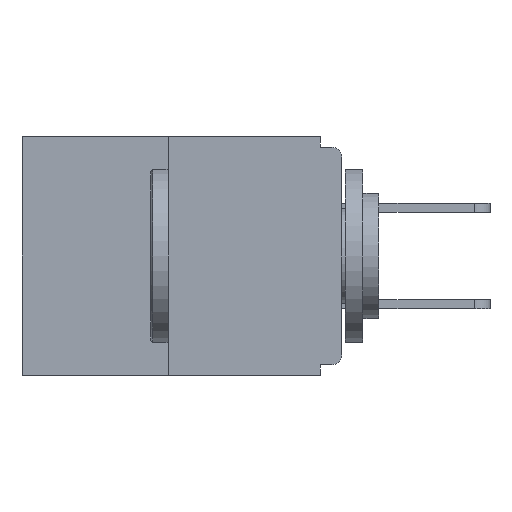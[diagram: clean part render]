
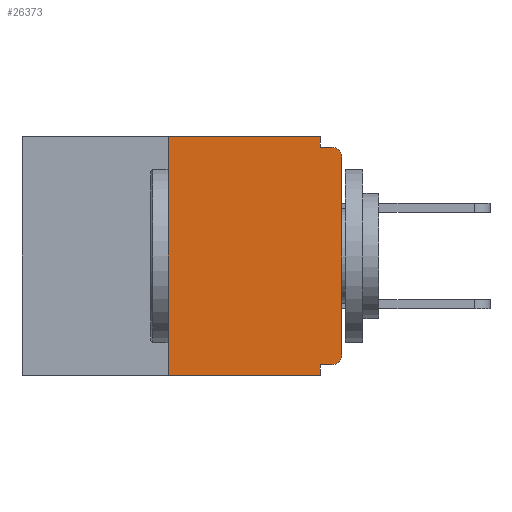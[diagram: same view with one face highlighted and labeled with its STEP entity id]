
A CAD part, left-side view. The second image highlights one B-rep face of the part: STEP entity #26373.
In plain terms, the highlighted planar face has unit normal (-1, 0, 0).
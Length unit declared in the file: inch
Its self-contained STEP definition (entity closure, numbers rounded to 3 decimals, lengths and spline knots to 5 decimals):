
#136 = CARTESIAN_POINT ( 'NONE',  ( 0., 0.031, -0.343 ) ) ;
#201 = CARTESIAN_POINT ( 'NONE',  ( 0., 0.46, 0. ) ) ;
#247 = CIRCLE ( 'NONE', #14551, 0.015 ) ;
#521 = ORIENTED_EDGE ( 'NONE', *, *, #13387, .T. ) ;
#748 = VERTEX_POINT ( 'NONE', #10406 ) ;
#1511 = DIRECTION ( 'NONE',  ( 0., -1., 0. ) ) ;
#1927 = VERTEX_POINT ( 'NONE', #22366 ) ;
#1938 = ORIENTED_EDGE ( 'NONE', *, *, #20720, .T. ) ;
#2018 = VECTOR ( 'NONE', #21718, 39.37008 ) ;
#2052 = LINE ( 'NONE', #16138, #20815 ) ;
#2487 = EDGE_CURVE ( 'NONE', #14383, #1927, #14177, .T. ) ;
#2576 = VERTEX_POINT ( 'NONE', #16046 ) ;
#2694 = ORIENTED_EDGE ( 'NONE', *, *, #5131, .F. ) ;
#2847 = CARTESIAN_POINT ( 'NONE',  ( 0., 0.015, -0.328 ) ) ;
#3844 = DIRECTION ( 'NONE',  ( 0., -1., 0. ) ) ;
#4310 = CARTESIAN_POINT ( 'NONE',  ( 0., 0.46, 0. ) ) ;
#4387 = LINE ( 'NONE', #22350, #19193 ) ;
#4426 = CARTESIAN_POINT ( 'NONE',  ( 0., 0.031, 0. ) ) ;
#5131 = EDGE_CURVE ( 'NONE', #22910, #2576, #16025, .T. ) ;
#5348 = DIRECTION ( 'NONE',  ( -1., 0., 0. ) ) ;
#5556 = CARTESIAN_POINT ( 'NONE',  ( 0., 0.015, -0.03 ) ) ;
#5672 = EDGE_LOOP ( 'NONE', ( #23078, #17036, #1938, #14433, #23446, #25387, #521, #17475, #18691, #2694 ) ) ;
#5759 = DIRECTION ( 'NONE',  ( -1., 0., 0. ) ) ;
#5862 = CARTESIAN_POINT ( 'NONE',  ( 0., 0.46, -0.343 ) ) ;
#6143 = CARTESIAN_POINT ( 'NONE',  ( 0., 0.25, 0. ) ) ;
#6789 = EDGE_CURVE ( 'NONE', #8303, #18234, #25096, .T. ) ;
#8303 = VERTEX_POINT ( 'NONE', #19210 ) ;
#8489 = DIRECTION ( 'NONE',  ( 0., 0., -1. ) ) ;
#8559 = DIRECTION ( 'NONE',  ( 0., 0., 1. ) ) ;
#8616 = VECTOR ( 'NONE', #8559, 39.37008 ) ;
#8622 = VERTEX_POINT ( 'NONE', #14036 ) ;
#9369 = VERTEX_POINT ( 'NONE', #2847 ) ;
#10406 = CARTESIAN_POINT ( 'NONE',  ( 0., 0.031, -0.328 ) ) ;
#11042 = LINE ( 'NONE', #26883, #14306 ) ;
#11385 = FACE_OUTER_BOUND ( 'NONE', #5672, .T. ) ;
#11930 = AXIS2_PLACEMENT_3D ( 'NONE', #201, #12721, #18848 ) ;
#12286 = VECTOR ( 'NONE', #3844, 39.37008 ) ;
#12721 = DIRECTION ( 'NONE',  ( 1., 0., 0. ) ) ;
#13387 = EDGE_CURVE ( 'NONE', #8622, #8303, #11042, .T. ) ;
#14036 = CARTESIAN_POINT ( 'NONE',  ( 0., 0., -0.313 ) ) ;
#14177 = LINE ( 'NONE', #6143, #8616 ) ;
#14306 = VECTOR ( 'NONE', #26518, 39.37008 ) ;
#14383 = VERTEX_POINT ( 'NONE', #14476 ) ;
#14433 = ORIENTED_EDGE ( 'NONE', *, *, #21808, .F. ) ;
#14476 = CARTESIAN_POINT ( 'NONE',  ( 0., 0.25, -0.343 ) ) ;
#14551 = AXIS2_PLACEMENT_3D ( 'NONE', #17958, #5348, #22087 ) ;
#15475 = LINE ( 'NONE', #4310, #26006 ) ;
#15816 = EDGE_CURVE ( 'NONE', #9369, #748, #16798, .T. ) ;
#16025 = LINE ( 'NONE', #4426, #24925 ) ;
#16046 = CARTESIAN_POINT ( 'NONE',  ( 0., 0.031, -0.015 ) ) ;
#16138 = CARTESIAN_POINT ( 'NONE',  ( 0., 0.031, -0.343 ) ) ;
#16158 = VERTEX_POINT ( 'NONE', #136 ) ;
#16798 = LINE ( 'NONE', #17321, #2018 ) ;
#17036 = ORIENTED_EDGE ( 'NONE', *, *, #2487, .F. ) ;
#17279 = DIRECTION ( 'NONE',  ( 0., -1., 0. ) ) ;
#17310 = AXIS2_PLACEMENT_3D ( 'NONE', #5556, #5759, #22383 ) ;
#17321 = CARTESIAN_POINT ( 'NONE',  ( 0., 0., -0.328 ) ) ;
#17475 = ORIENTED_EDGE ( 'NONE', *, *, #6789, .T. ) ;
#17958 = CARTESIAN_POINT ( 'NONE',  ( 0., 0.015, -0.313 ) ) ;
#18234 = VERTEX_POINT ( 'NONE', #20882 ) ;
#18323 = EDGE_CURVE ( 'NONE', #9369, #8622, #247, .T. ) ;
#18691 = ORIENTED_EDGE ( 'NONE', *, *, #20462, .F. ) ;
#18848 = DIRECTION ( 'NONE',  ( 0., 0., -1. ) ) ;
#19193 = VECTOR ( 'NONE', #1511, 39.37008 ) ;
#19210 = CARTESIAN_POINT ( 'NONE',  ( 0., 0., -0.03 ) ) ;
#20406 = DIRECTION ( 'NONE',  ( 0., 0., -1. ) ) ;
#20462 = EDGE_CURVE ( 'NONE', #2576, #18234, #4387, .T. ) ;
#20720 = EDGE_CURVE ( 'NONE', #14383, #16158, #23788, .T. ) ;
#20815 = VECTOR ( 'NONE', #20406, 39.37008 ) ;
#20882 = CARTESIAN_POINT ( 'NONE',  ( 0., 0.015, -0.015 ) ) ;
#21718 = DIRECTION ( 'NONE',  ( 0., 1., 0. ) ) ;
#21808 = EDGE_CURVE ( 'NONE', #748, #16158, #2052, .T. ) ;
#22087 = DIRECTION ( 'NONE',  ( 0., 0., -1. ) ) ;
#22350 = CARTESIAN_POINT ( 'NONE',  ( 0., 0., -0.015 ) ) ;
#22366 = CARTESIAN_POINT ( 'NONE',  ( 0., 0.25, 0. ) ) ;
#22383 = DIRECTION ( 'NONE',  ( 0., 0., -1. ) ) ;
#22910 = VERTEX_POINT ( 'NONE', #22912 ) ;
#22912 = CARTESIAN_POINT ( 'NONE',  ( 0., 0.031, 0. ) ) ;
#23078 = ORIENTED_EDGE ( 'NONE', *, *, #25336, .F. ) ;
#23446 = ORIENTED_EDGE ( 'NONE', *, *, #15816, .F. ) ;
#23788 = LINE ( 'NONE', #5862, #12286 ) ;
#24925 = VECTOR ( 'NONE', #8489, 39.37008 ) ;
#25096 = CIRCLE ( 'NONE', #17310, 0.015 ) ;
#25285 = PLANE ( 'NONE',  #11930 ) ;
#25336 = EDGE_CURVE ( 'NONE', #1927, #22910, #15475, .T. ) ;
#25387 = ORIENTED_EDGE ( 'NONE', *, *, #18323, .T. ) ;
#26006 = VECTOR ( 'NONE', #17279, 39.37008 ) ;
#26373 = ADVANCED_FACE ( 'NONE', ( #11385 ), #25285, .F. ) ;
#26518 = DIRECTION ( 'NONE',  ( 0., 0., 1. ) ) ;
#26883 = CARTESIAN_POINT ( 'NONE',  ( 0., 0., 0. ) ) ;
